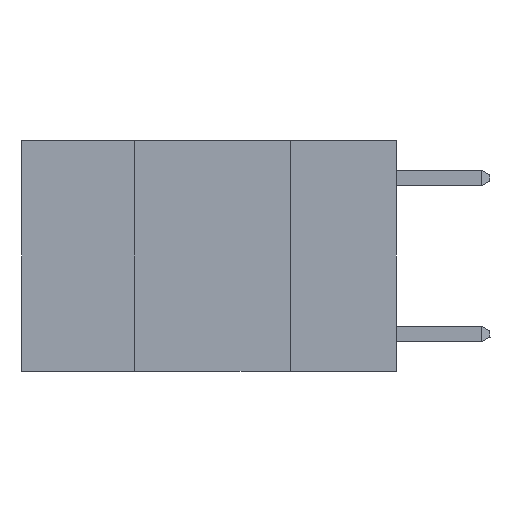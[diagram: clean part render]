
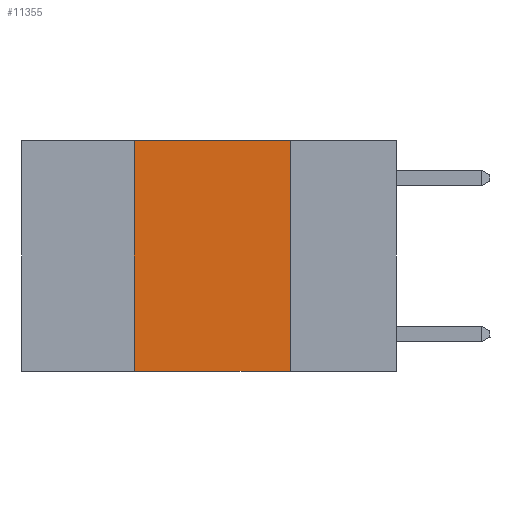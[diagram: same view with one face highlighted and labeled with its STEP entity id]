
A CAD part, left-side view. The second image highlights one B-rep face of the part: STEP entity #11355.
In plain terms, the highlighted planar face has unit normal (-1, 0, 0).
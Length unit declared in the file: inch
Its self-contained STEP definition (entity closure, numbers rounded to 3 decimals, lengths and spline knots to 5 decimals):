
#152 = VERTEX_POINT ( 'NONE', #11533 ) ;
#516 = CARTESIAN_POINT ( 'NONE',  ( 0., 0.42, -0.37 ) ) ;
#740 = LINE ( 'NONE', #11959, #12966 ) ;
#1488 = DIRECTION ( 'NONE',  ( 1., 0., 0. ) ) ;
#2396 = ORIENTED_EDGE ( 'NONE', *, *, #13758, .F. ) ;
#2655 = VERTEX_POINT ( 'NONE', #13840 ) ;
#3952 = ORIENTED_EDGE ( 'NONE', *, *, #5193, .T. ) ;
#5193 = EDGE_CURVE ( 'NONE', #9596, #152, #6615, .T. ) ;
#5672 = FACE_OUTER_BOUND ( 'NONE', #6705, .T. ) ;
#5877 = VECTOR ( 'NONE', #14025, 39.37008 ) ;
#6072 = DIRECTION ( 'NONE',  ( 0., 0., -1. ) ) ;
#6138 = LINE ( 'NONE', #10143, #12040 ) ;
#6226 = AXIS2_PLACEMENT_3D ( 'NONE', #12114, #1488, #9817 ) ;
#6615 = LINE ( 'NONE', #12880, #5877 ) ;
#6705 = EDGE_LOOP ( 'NONE', ( #2396, #14375, #12230, #3952 ) ) ;
#7432 = PLANE ( 'NONE',  #6226 ) ;
#9596 = VERTEX_POINT ( 'NONE', #516 ) ;
#9817 = DIRECTION ( 'NONE',  ( 0., 0., -1. ) ) ;
#10143 = CARTESIAN_POINT ( 'NONE',  ( 0., 0.42, 0. ) ) ;
#10524 = CARTESIAN_POINT ( 'NONE',  ( 0., 0.6, 0. ) ) ;
#11355 = ADVANCED_FACE ( 'NONE', ( #5672 ), #7432, .F. ) ;
#11533 = CARTESIAN_POINT ( 'NONE',  ( 0., 0.17, -0.37 ) ) ;
#11696 = DIRECTION ( 'NONE',  ( 0., -1., 0. ) ) ;
#11959 = CARTESIAN_POINT ( 'NONE',  ( 0., 0.17, 0. ) ) ;
#12040 = VECTOR ( 'NONE', #12466, 39.37008 ) ;
#12114 = CARTESIAN_POINT ( 'NONE',  ( 0., 0.6, 0. ) ) ;
#12220 = LINE ( 'NONE', #10524, #14923 ) ;
#12230 = ORIENTED_EDGE ( 'NONE', *, *, #14679, .F. ) ;
#12466 = DIRECTION ( 'NONE',  ( 0., 0., 1. ) ) ;
#12880 = CARTESIAN_POINT ( 'NONE',  ( 0., 0.6, -0.37 ) ) ;
#12966 = VECTOR ( 'NONE', #6072, 39.37008 ) ;
#13758 = EDGE_CURVE ( 'NONE', #14727, #152, #740, .T. ) ;
#13840 = CARTESIAN_POINT ( 'NONE',  ( 0., 0.42, 0. ) ) ;
#14025 = DIRECTION ( 'NONE',  ( 0., -1., 0. ) ) ;
#14247 = EDGE_CURVE ( 'NONE', #2655, #14727, #12220, .T. ) ;
#14375 = ORIENTED_EDGE ( 'NONE', *, *, #14247, .F. ) ;
#14679 = EDGE_CURVE ( 'NONE', #9596, #2655, #6138, .T. ) ;
#14727 = VERTEX_POINT ( 'NONE', #14837 ) ;
#14837 = CARTESIAN_POINT ( 'NONE',  ( 0., 0.17, 0. ) ) ;
#14923 = VECTOR ( 'NONE', #11696, 39.37008 ) ;
